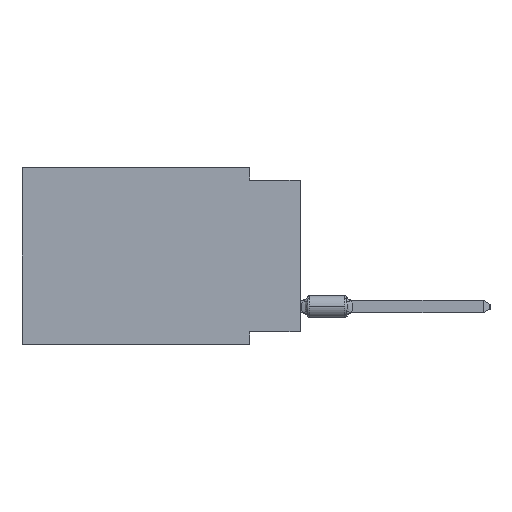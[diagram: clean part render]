
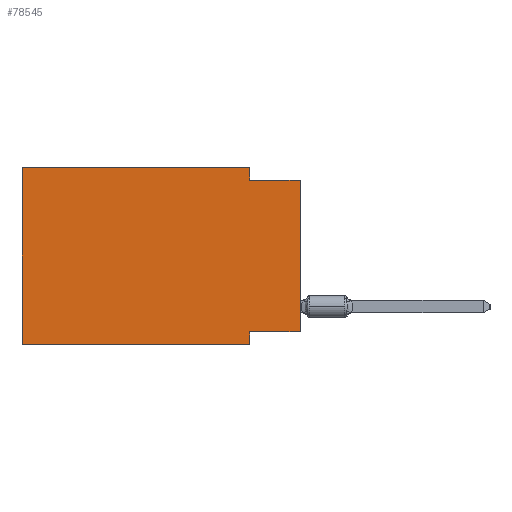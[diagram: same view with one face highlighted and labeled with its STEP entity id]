
A CAD part, left-side view. The second image highlights one B-rep face of the part: STEP entity #78545.
In plain terms, the highlighted planar face has unit normal (-1, 0, 0).
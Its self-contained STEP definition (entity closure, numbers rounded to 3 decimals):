
#165 = EDGE_CURVE ( 'NONE', #35267, #30312, #51653, .T. ) ;
#2609 = ORIENTED_EDGE ( 'NONE', *, *, #65010, .F. ) ;
#3268 = CARTESIAN_POINT ( 'NONE',  ( 0., 0., -8.255 ) ) ;
#3670 = DIRECTION ( 'NONE',  ( 1., 0., 0. ) ) ;
#5167 = CARTESIAN_POINT ( 'NONE',  ( 0., 13.97, 0. ) ) ;
#7438 = VECTOR ( 'NONE', #45683, 1000. ) ;
#7939 = LINE ( 'NONE', #22116, #24718 ) ;
#8123 = VERTEX_POINT ( 'NONE', #3268 ) ;
#13961 = EDGE_LOOP ( 'NONE', ( #52640, #2609, #77715, #14189, #14178, #84059, #35866, #85902 ) ) ;
#14178 = ORIENTED_EDGE ( 'NONE', *, *, #165, .F. ) ;
#14189 = ORIENTED_EDGE ( 'NONE', *, *, #29100, .F. ) ;
#17364 = CARTESIAN_POINT ( 'NONE',  ( 0., 13.97, 0. ) ) ;
#21537 = EDGE_CURVE ( 'NONE', #35267, #77885, #85437, .T. ) ;
#21686 = VECTOR ( 'NONE', #67549, 1000. ) ;
#22116 = CARTESIAN_POINT ( 'NONE',  ( 0., 0., 0. ) ) ;
#24081 = CARTESIAN_POINT ( 'NONE',  ( 0., 2.54, -8.255 ) ) ;
#24718 = VECTOR ( 'NONE', #74356, 1000. ) ;
#29100 = EDGE_CURVE ( 'NONE', #30312, #39370, #63948, .T. ) ;
#29728 = EDGE_CURVE ( 'NONE', #39370, #64617, #82791, .T. ) ;
#30312 = VERTEX_POINT ( 'NONE', #5167 ) ;
#30579 = EDGE_CURVE ( 'NONE', #8123, #63989, #7939, .T. ) ;
#31762 = LINE ( 'NONE', #84496, #43881 ) ;
#32995 = FACE_OUTER_BOUND ( 'NONE', #13961, .T. ) ;
#35267 = VERTEX_POINT ( 'NONE', #66171 ) ;
#35866 = ORIENTED_EDGE ( 'NONE', *, *, #53561, .F. ) ;
#36994 = CARTESIAN_POINT ( 'NONE',  ( 0., 13.97, 0. ) ) ;
#38441 = AXIS2_PLACEMENT_3D ( 'NONE', #17364, #3670, #63742 ) ;
#38527 = VECTOR ( 'NONE', #56131, 1000. ) ;
#39370 = VERTEX_POINT ( 'NONE', #82034 ) ;
#43881 = VECTOR ( 'NONE', #52772, 1000. ) ;
#45683 = DIRECTION ( 'NONE',  ( 0., 0., -1. ) ) ;
#46790 = CARTESIAN_POINT ( 'NONE',  ( 0., 2.54, -8.89 ) ) ;
#50478 = CARTESIAN_POINT ( 'NONE',  ( 0., 0., -0.635 ) ) ;
#51653 = LINE ( 'NONE', #36994, #54781 ) ;
#52640 = ORIENTED_EDGE ( 'NONE', *, *, #30579, .T. ) ;
#52772 = DIRECTION ( 'NONE',  ( 0., 0., -1. ) ) ;
#53561 = EDGE_CURVE ( 'NONE', #54970, #77885, #31762, .T. ) ;
#54405 = CARTESIAN_POINT ( 'NONE',  ( 0., 0., -8.255 ) ) ;
#54473 = PLANE ( 'NONE',  #38441 ) ;
#54781 = VECTOR ( 'NONE', #81440, 1000. ) ;
#54970 = VERTEX_POINT ( 'NONE', #24081 ) ;
#55651 = DIRECTION ( 'NONE',  ( 0., -1., 0. ) ) ;
#56131 = DIRECTION ( 'NONE',  ( 0., -1., 0. ) ) ;
#57809 = LINE ( 'NONE', #50478, #21686 ) ;
#63742 = DIRECTION ( 'NONE',  ( 0., 0., -1. ) ) ;
#63948 = LINE ( 'NONE', #90463, #38527 ) ;
#63989 = VERTEX_POINT ( 'NONE', #69809 ) ;
#64617 = VERTEX_POINT ( 'NONE', #74486 ) ;
#65010 = EDGE_CURVE ( 'NONE', #64617, #63989, #57809, .T. ) ;
#66171 = CARTESIAN_POINT ( 'NONE',  ( 0., 13.97, -8.89 ) ) ;
#67549 = DIRECTION ( 'NONE',  ( 0., -1., 0. ) ) ;
#68580 = DIRECTION ( 'NONE',  ( 0., 1., 0. ) ) ;
#69809 = CARTESIAN_POINT ( 'NONE',  ( 0., 0., -0.635 ) ) ;
#72070 = VECTOR ( 'NONE', #55651, 1000. ) ;
#74356 = DIRECTION ( 'NONE',  ( 0., 0., 1. ) ) ;
#74486 = CARTESIAN_POINT ( 'NONE',  ( 0., 2.54, -0.635 ) ) ;
#77489 = EDGE_CURVE ( 'NONE', #8123, #54970, #90066, .T. ) ;
#77715 = ORIENTED_EDGE ( 'NONE', *, *, #29728, .F. ) ;
#77885 = VERTEX_POINT ( 'NONE', #46790 ) ;
#78545 = ADVANCED_FACE ( 'NONE', ( #32995 ), #54473, .F. ) ;
#80537 = VECTOR ( 'NONE', #68580, 1000. ) ;
#81440 = DIRECTION ( 'NONE',  ( 0., 0., 1. ) ) ;
#81829 = CARTESIAN_POINT ( 'NONE',  ( 0., 2.54, 0. ) ) ;
#82034 = CARTESIAN_POINT ( 'NONE',  ( 0., 2.54, 0. ) ) ;
#82791 = LINE ( 'NONE', #81829, #7438 ) ;
#84059 = ORIENTED_EDGE ( 'NONE', *, *, #21537, .T. ) ;
#84496 = CARTESIAN_POINT ( 'NONE',  ( 0., 2.54, -8.89 ) ) ;
#85437 = LINE ( 'NONE', #86398, #72070 ) ;
#85902 = ORIENTED_EDGE ( 'NONE', *, *, #77489, .F. ) ;
#86398 = CARTESIAN_POINT ( 'NONE',  ( 0., 13.97, -8.89 ) ) ;
#90066 = LINE ( 'NONE', #54405, #80537 ) ;
#90463 = CARTESIAN_POINT ( 'NONE',  ( 0., 13.97, 0. ) ) ;
